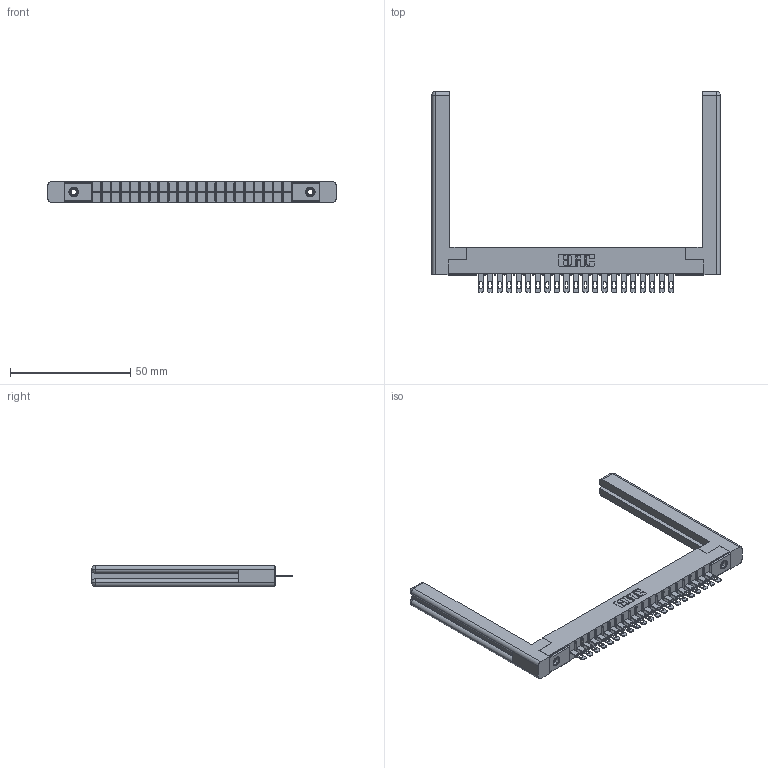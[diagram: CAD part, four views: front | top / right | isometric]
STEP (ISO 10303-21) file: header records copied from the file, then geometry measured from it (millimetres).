
FILE_DESCRIPTION (( 'STEP AP203' ), '1' );
FILE_NAME ('356-021-500-158.STEP', '2018-08-01T19:46:53', ( '' ), ( '' ), 'SwSTEP 2.0', 'SolidWorks 2016', '' );
FILE_SCHEMA (( 'CONFIG_CONTROL_DESIGN' ));
Length unit declared in the file: inch
Products named in the file (5): 306-290-001_100; 345-250-001_345-250-001-102; 307-220-058; 356-021-500-158; 306 Part_.156 Dia
Assembly tree (26 placements, depth 2):
  356-021-500-158
    306 Part_.156 Dia
    306-290-001_100  x21
    345-250-001_345-250-001-102  x2
    307-220-058  x2
Bounding box: 119.84 x 83.52 x 8.71 mm (x, y, z)
Volume: 15901.1 mm3; surface area: 17807.8 mm2
Topology: 26 solids, 26 shells, 1854 faces, 5185 edges, 3330 vertices
Faces by surface type: plane 1202, cylinder 544, sphere 84, cone 12, torus 12
Entity records: 25101 total; most frequent: CARTESIAN_POINT 4221, ORIENTED_EDGE 4124, DIRECTION 4120, EDGE_CURVE 2062, VECTOR 1594, LINE 1594, VERTEX_POINT 1310, AXIS2_PLACEMENT_3D 1263
